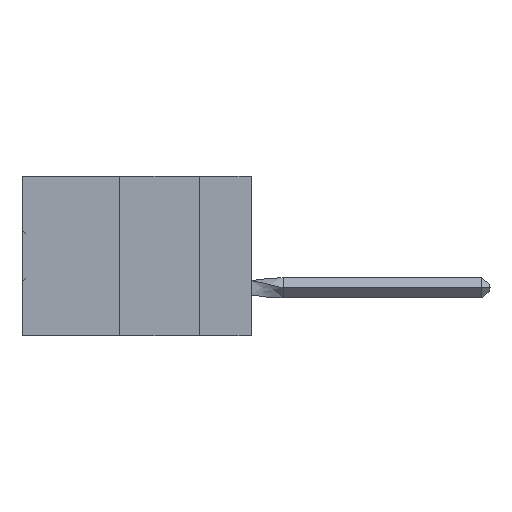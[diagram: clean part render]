
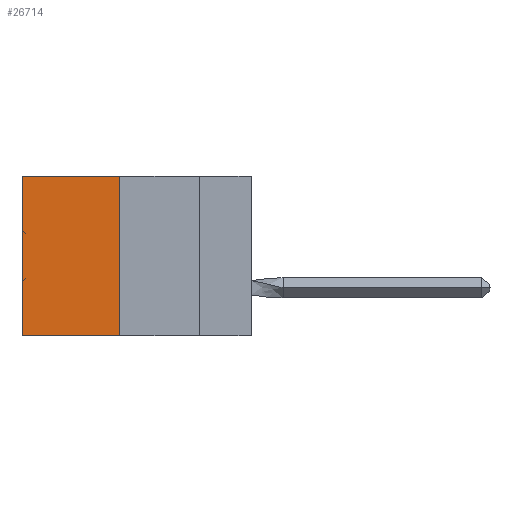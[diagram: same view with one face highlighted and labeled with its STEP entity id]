
A CAD part, left-side view. The second image highlights one B-rep face of the part: STEP entity #26714.
In plain terms, the highlighted planar face has unit normal (-1, 0, 0).
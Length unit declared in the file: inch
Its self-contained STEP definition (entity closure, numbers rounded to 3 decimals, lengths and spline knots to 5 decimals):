
#801 = EDGE_CURVE ( 'NONE', #16509, #19352, #13219, .T. ) ;
#1917 = PLANE ( 'NONE',  #35972 ) ;
#2115 = DIRECTION ( 'NONE',  ( 0., 0., -1. ) ) ;
#2770 = DIRECTION ( 'NONE',  ( 0., 0., -1. ) ) ;
#4064 = EDGE_CURVE ( 'NONE', #49618, #19352, #37301, .T. ) ;
#4198 = DIRECTION ( 'NONE',  ( 0., 0., -1. ) ) ;
#4626 = DIRECTION ( 'NONE',  ( 0., 1., 0. ) ) ;
#6747 = CARTESIAN_POINT ( 'NONE',  ( 0.305, 0.413, -0.5 ) ) ;
#7057 = DIRECTION ( 'NONE',  ( 0., 1., 0. ) ) ;
#10155 = LINE ( 'NONE', #11620, #61122 ) ;
#11620 = CARTESIAN_POINT ( 'NONE',  ( 0.305, 0.413, -0.5 ) ) ;
#13219 = LINE ( 'NONE', #41305, #19900 ) ;
#16509 = VERTEX_POINT ( 'NONE', #41688 ) ;
#17184 = FACE_OUTER_BOUND ( 'NONE', #34895, .T. ) ;
#19352 = VERTEX_POINT ( 'NONE', #35687 ) ;
#19900 = VECTOR ( 'NONE', #7057, 39.37008 ) ;
#19997 = CARTESIAN_POINT ( 'NONE',  ( 0.305, 0.72, 0. ) ) ;
#21985 = ORIENTED_EDGE ( 'NONE', *, *, #4064, .T. ) ;
#26714 = ADVANCED_FACE ( 'NONE', ( #17184 ), #1917, .F. ) ;
#28231 = CARTESIAN_POINT ( 'NONE',  ( 0.305, 0.72, -0.5 ) ) ;
#34895 = EDGE_LOOP ( 'NONE', ( #21985, #60707, #47693, #59098 ) ) ;
#35687 = CARTESIAN_POINT ( 'NONE',  ( 0.305, 0.72, -0.5 ) ) ;
#35972 = AXIS2_PLACEMENT_3D ( 'NONE', #6747, #44824, #2115 ) ;
#37301 = LINE ( 'NONE', #28231, #60668 ) ;
#37410 = CARTESIAN_POINT ( 'NONE',  ( 0.305, 0.413, 0. ) ) ;
#38028 = CARTESIAN_POINT ( 'NONE',  ( 0.305, 0.413, 0. ) ) ;
#41305 = CARTESIAN_POINT ( 'NONE',  ( 0.305, 0.413, -0.5 ) ) ;
#41688 = CARTESIAN_POINT ( 'NONE',  ( 0.305, 0.413, -0.5 ) ) ;
#44824 = DIRECTION ( 'NONE',  ( 1., 0., 0. ) ) ;
#47527 = LINE ( 'NONE', #38028, #56493 ) ;
#47693 = ORIENTED_EDGE ( 'NONE', *, *, #51391, .F. ) ;
#49618 = VERTEX_POINT ( 'NONE', #19997 ) ;
#51391 = EDGE_CURVE ( 'NONE', #59799, #16509, #10155, .T. ) ;
#51693 = EDGE_CURVE ( 'NONE', #59799, #49618, #47527, .T. ) ;
#56493 = VECTOR ( 'NONE', #4626, 39.37008 ) ;
#59098 = ORIENTED_EDGE ( 'NONE', *, *, #51693, .T. ) ;
#59799 = VERTEX_POINT ( 'NONE', #37410 ) ;
#60668 = VECTOR ( 'NONE', #4198, 39.37008 ) ;
#60707 = ORIENTED_EDGE ( 'NONE', *, *, #801, .F. ) ;
#61122 = VECTOR ( 'NONE', #2770, 39.37008 ) ;
